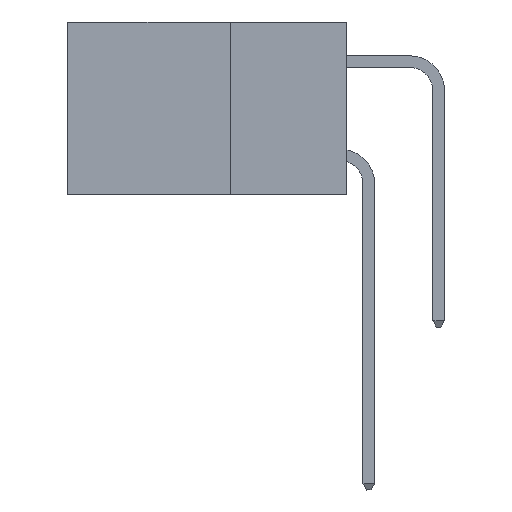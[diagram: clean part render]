
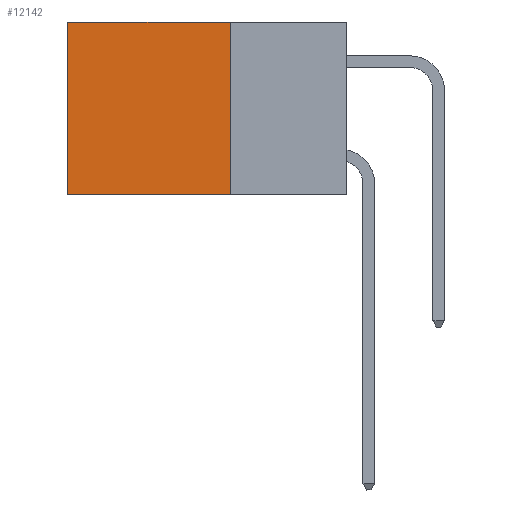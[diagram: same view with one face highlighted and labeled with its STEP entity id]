
A CAD part, left-side view. The second image highlights one B-rep face of the part: STEP entity #12142.
In plain terms, the highlighted planar face has unit normal (-1, 0, 0).
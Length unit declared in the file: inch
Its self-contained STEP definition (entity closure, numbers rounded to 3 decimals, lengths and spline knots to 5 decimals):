
#1774 = EDGE_CURVE ( 'NONE', #15017, #20342, #12818, .T. ) ;
#2029 = CARTESIAN_POINT ( 'NONE',  ( 0.2875, 0.25, 0. ) ) ;
#2120 = VECTOR ( 'NONE', #9216, 39.37008 ) ;
#4797 = CARTESIAN_POINT ( 'NONE',  ( 0.2875, 0.25, -0.37 ) ) ;
#5448 = PLANE ( 'NONE',  #27416 ) ;
#5769 = LINE ( 'NONE', #23758, #2120 ) ;
#6869 = DIRECTION ( 'NONE',  ( 0., 0., -1. ) ) ;
#7031 = ORIENTED_EDGE ( 'NONE', *, *, #18232, .T. ) ;
#7554 = CARTESIAN_POINT ( 'NONE',  ( 0.2875, 0.6, 0. ) ) ;
#7751 = DIRECTION ( 'NONE',  ( 1., 0., 0. ) ) ;
#7809 = EDGE_CURVE ( 'NONE', #22584, #24180, #11074, .T. ) ;
#9216 = DIRECTION ( 'NONE',  ( 0., 1., 0. ) ) ;
#10047 = EDGE_CURVE ( 'NONE', #20342, #24180, #5769, .T. ) ;
#11063 = CARTESIAN_POINT ( 'NONE',  ( 0.2875, 0.6, -0.37 ) ) ;
#11074 = LINE ( 'NONE', #7554, #22681 ) ;
#11262 = EDGE_LOOP ( 'NONE', ( #23952, #18378, #12419, #7031 ) ) ;
#12142 = ADVANCED_FACE ( 'NONE', ( #25694 ), #5448, .F. ) ;
#12321 = CARTESIAN_POINT ( 'NONE',  ( 0.2875, 0.6, 0. ) ) ;
#12419 = ORIENTED_EDGE ( 'NONE', *, *, #1774, .F. ) ;
#12818 = LINE ( 'NONE', #2029, #16818 ) ;
#12919 = DIRECTION ( 'NONE',  ( 0., 1., 0. ) ) ;
#13698 = DIRECTION ( 'NONE',  ( 0., 0., -1. ) ) ;
#13919 = CARTESIAN_POINT ( 'NONE',  ( 0.2875, 0.25, 0. ) ) ;
#14492 = VECTOR ( 'NONE', #12919, 39.37008 ) ;
#15017 = VERTEX_POINT ( 'NONE', #15789 ) ;
#15789 = CARTESIAN_POINT ( 'NONE',  ( 0.2875, 0.25, 0. ) ) ;
#16818 = VECTOR ( 'NONE', #6869, 39.37008 ) ;
#18232 = EDGE_CURVE ( 'NONE', #15017, #22584, #20114, .T. ) ;
#18255 = DIRECTION ( 'NONE',  ( 0., 0., -1. ) ) ;
#18378 = ORIENTED_EDGE ( 'NONE', *, *, #10047, .F. ) ;
#20114 = LINE ( 'NONE', #27347, #14492 ) ;
#20342 = VERTEX_POINT ( 'NONE', #4797 ) ;
#22584 = VERTEX_POINT ( 'NONE', #12321 ) ;
#22681 = VECTOR ( 'NONE', #13698, 39.37008 ) ;
#23758 = CARTESIAN_POINT ( 'NONE',  ( 0.2875, 0.25, -0.37 ) ) ;
#23952 = ORIENTED_EDGE ( 'NONE', *, *, #7809, .T. ) ;
#24180 = VERTEX_POINT ( 'NONE', #11063 ) ;
#25694 = FACE_OUTER_BOUND ( 'NONE', #11262, .T. ) ;
#27347 = CARTESIAN_POINT ( 'NONE',  ( 0.2875, 0.25, 0. ) ) ;
#27416 = AXIS2_PLACEMENT_3D ( 'NONE', #13919, #7751, #18255 ) ;
